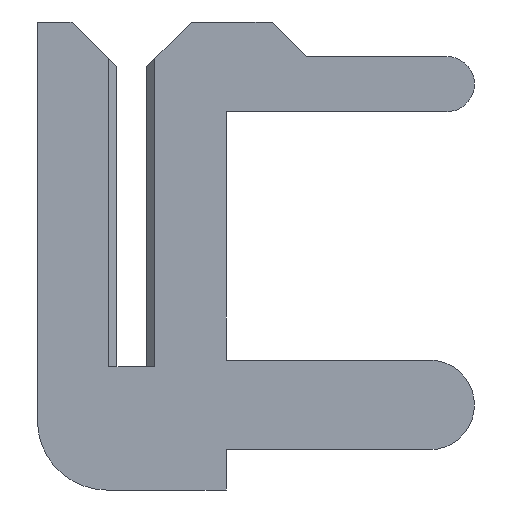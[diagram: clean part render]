
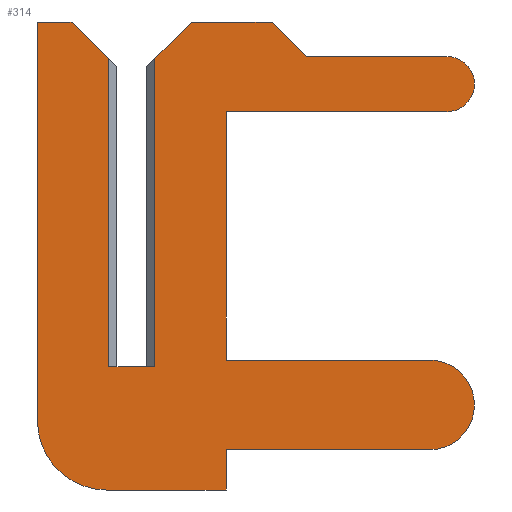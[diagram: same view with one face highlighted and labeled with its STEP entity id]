
A CAD part, left-side view. The second image highlights one B-rep face of the part: STEP entity #314.
In plain terms, the highlighted planar face has unit normal (-1, 0, 0).
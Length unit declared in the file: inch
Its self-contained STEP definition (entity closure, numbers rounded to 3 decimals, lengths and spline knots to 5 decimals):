
#5 = ORIENTED_EDGE ( 'NONE', *, *, #1200, .F. ) ;
#7 = VERTEX_POINT ( 'NONE', #64 ) ;
#8 = EDGE_CURVE ( 'NONE', #683, #844, #404, .T. ) ;
#40 = VECTOR ( 'NONE', #839, 39.37008 ) ;
#43 = AXIS2_PLACEMENT_3D ( 'NONE', #395, #286, #94 ) ;
#48 = CARTESIAN_POINT ( 'NONE',  ( -0.01, -0.137, 0.111 ) ) ;
#51 = VERTEX_POINT ( 'NONE', #527 ) ;
#52 = EDGE_CURVE ( 'NONE', #713, #859, #476, .T. ) ;
#58 = DIRECTION ( 'NONE',  ( 0., 0., 1. ) ) ;
#59 = VERTEX_POINT ( 'NONE', #336 ) ;
#64 = CARTESIAN_POINT ( 'NONE',  ( -0.01, -0.01, 0. ) ) ;
#67 = EDGE_CURVE ( 'NONE', #59, #7, #883, .T. ) ;
#69 = CARTESIAN_POINT ( 'NONE',  ( -0.01, -0.1295, 0.003 ) ) ;
#86 = LINE ( 'NONE', #69, #1009 ) ;
#94 = DIRECTION ( 'NONE',  ( 0., 0., 1. ) ) ;
#118 = EDGE_LOOP ( 'NONE', ( #1059, #1040, #791, #230, #5, #1042, #881, #497, #1221, #818, #893, #371, #251, #534, #278, #431, #1159, #1102, #756 ) ) ;
#146 = CARTESIAN_POINT ( 'NONE',  ( -0.01, -0.041, 0.111 ) ) ;
#148 = AXIS2_PLACEMENT_3D ( 'NONE', #1144, #942, #1112 ) ;
#156 = EDGE_CURVE ( 'NONE', #859, #778, #1106, .T. ) ;
#180 = CARTESIAN_POINT ( 'NONE',  ( -0.01, -0.041, -0.0535 ) ) ;
#208 = EDGE_CURVE ( 'NONE', #774, #328, #1032, .T. ) ;
#223 = VECTOR ( 'NONE', #699, 39.37008 ) ;
#230 = ORIENTED_EDGE ( 'NONE', *, *, #208, .T. ) ;
#237 = VECTOR ( 'NONE', #835, 39.37008 ) ;
#246 = VECTOR ( 'NONE', #58, 39.37008 ) ;
#251 = ORIENTED_EDGE ( 'NONE', *, *, #941, .F. ) ;
#257 = DIRECTION ( 'NONE',  ( 0., 0., 1. ) ) ;
#278 = ORIENTED_EDGE ( 'NONE', *, *, #156, .F. ) ;
#284 = CARTESIAN_POINT ( 'NONE',  ( -0.01, -0.041, 0.003 ) ) ;
#286 = DIRECTION ( 'NONE',  ( 1., 0., 0. ) ) ;
#287 = EDGE_CURVE ( 'NONE', #59, #1206, #653, .T. ) ;
#288 = CARTESIAN_POINT ( 'NONE',  ( -0.01, 0.0065, 0.1305 ) ) ;
#294 = VERTEX_POINT ( 'NONE', #284 ) ;
#307 = DIRECTION ( 'NONE',  ( 0., -1., 0. ) ) ;
#314 = ADVANCED_FACE ( 'NONE', ( #885 ), #937, .T. ) ;
#325 = CARTESIAN_POINT ( 'NONE',  ( -0.01, 0.0065, 0. ) ) ;
#328 = VERTEX_POINT ( 'NONE', #1034 ) ;
#333 = CARTESIAN_POINT ( 'NONE',  ( -0.01, 0.01, 0. ) ) ;
#336 = CARTESIAN_POINT ( 'NONE',  ( -0.01, -0.01, 0.134 ) ) ;
#346 = DIRECTION ( 'NONE',  ( 0., 0., -1. ) ) ;
#371 = ORIENTED_EDGE ( 'NONE', *, *, #519, .F. ) ;
#382 = DIRECTION ( 'NONE',  ( 0., -1., 0. ) ) ;
#395 = CARTESIAN_POINT ( 'NONE',  ( -0.01, -0.1295, -0.0165 ) ) ;
#404 = CIRCLE ( 'NONE', #1037, 0.03 ) ;
#419 = DIRECTION ( 'NONE',  ( 0., -1., 0. ) ) ;
#431 = ORIENTED_EDGE ( 'NONE', *, *, #52, .F. ) ;
#432 = CARTESIAN_POINT ( 'NONE',  ( -0.01, 0.011, -0.0235 ) ) ;
#433 = DIRECTION ( 'NONE',  ( 0., -1., 0. ) ) ;
#440 = CIRCLE ( 'NONE', #43, 0.0195 ) ;
#442 = CARTESIAN_POINT ( 'NONE',  ( -0.01, 0.041, 0.15 ) ) ;
#452 = EDGE_CURVE ( 'NONE', #680, #651, #915, .T. ) ;
#476 = CIRCLE ( 'NONE', #506, 0.012 ) ;
#482 = VECTOR ( 'NONE', #1038, 39.37008 ) ;
#483 = CARTESIAN_POINT ( 'NONE',  ( -0.01, -0.076, 0.135 ) ) ;
#485 = LINE ( 'NONE', #1148, #913 ) ;
#492 = LINE ( 'NONE', #442, #246 ) ;
#494 = VERTEX_POINT ( 'NONE', #975 ) ;
#497 = ORIENTED_EDGE ( 'NONE', *, *, #8, .F. ) ;
#506 = AXIS2_PLACEMENT_3D ( 'NONE', #716, #812, #257 ) ;
#519 = EDGE_CURVE ( 'NONE', #730, #51, #440, .T. ) ;
#520 = DIRECTION ( 'NONE',  ( 1., 0., 0. ) ) ;
#521 = CARTESIAN_POINT ( 'NONE',  ( -0.01, 0.041, -0.0235 ) ) ;
#525 = VERTEX_POINT ( 'NONE', #1132 ) ;
#527 = CARTESIAN_POINT ( 'NONE',  ( -0.01, -0.1295, -0.036 ) ) ;
#531 = CARTESIAN_POINT ( 'NONE',  ( -0.01, 0.026, 0.15 ) ) ;
#534 = ORIENTED_EDGE ( 'NONE', *, *, #599, .F. ) ;
#535 = VERTEX_POINT ( 'NONE', #1125 ) ;
#542 = LINE ( 'NONE', #858, #886 ) ;
#552 = LINE ( 'NONE', #180, #40 ) ;
#577 = CARTESIAN_POINT ( 'NONE',  ( -0.01, 0.011, -0.0535 ) ) ;
#591 = EDGE_CURVE ( 'NONE', #525, #683, #485, .T. ) ;
#599 = EDGE_CURVE ( 'NONE', #778, #294, #641, .T. ) ;
#611 = CARTESIAN_POINT ( 'NONE',  ( -0.01, -0.137, 0.135 ) ) ;
#632 = EDGE_CURVE ( 'NONE', #651, #713, #542, .T. ) ;
#641 = LINE ( 'NONE', #765, #869 ) ;
#651 = VERTEX_POINT ( 'NONE', #483 ) ;
#653 = LINE ( 'NONE', #1130, #482 ) ;
#665 = CARTESIAN_POINT ( 'NONE',  ( -0.01, -0.026, 0.15 ) ) ;
#670 = DIRECTION ( 'NONE',  ( 0., -0.707, -0.707 ) ) ;
#680 = VERTEX_POINT ( 'NONE', #1060 ) ;
#681 = EDGE_CURVE ( 'NONE', #1206, #680, #1070, .T. ) ;
#683 = VERTEX_POINT ( 'NONE', #577 ) ;
#686 = DIRECTION ( 'NONE',  ( 0., -0.707, -0.707 ) ) ;
#698 = CARTESIAN_POINT ( 'NONE',  ( -0.01, -0.076, 0.135 ) ) ;
#699 = DIRECTION ( 'NONE',  ( 0., 1., 0. ) ) ;
#704 = CARTESIAN_POINT ( 'NONE',  ( -0.01, -0.041, -0.036 ) ) ;
#707 = VECTOR ( 'NONE', #433, 39.37008 ) ;
#713 = VERTEX_POINT ( 'NONE', #611 ) ;
#716 = CARTESIAN_POINT ( 'NONE',  ( -0.01, -0.137, 0.123 ) ) ;
#723 = VERTEX_POINT ( 'NONE', #1185 ) ;
#730 = VERTEX_POINT ( 'NONE', #994 ) ;
#733 = CARTESIAN_POINT ( 'NONE',  ( -0.01, 0.01, -0.0235 ) ) ;
#736 = VECTOR ( 'NONE', #686, 39.37008 ) ;
#749 = EDGE_CURVE ( 'NONE', #51, #723, #973, .T. ) ;
#756 = ORIENTED_EDGE ( 'NONE', *, *, #681, .F. ) ;
#765 = CARTESIAN_POINT ( 'NONE',  ( -0.01, -0.041, 0.003 ) ) ;
#774 = VERTEX_POINT ( 'NONE', #333 ) ;
#778 = VERTEX_POINT ( 'NONE', #146 ) ;
#789 = VECTOR ( 'NONE', #346, 39.37008 ) ;
#791 = ORIENTED_EDGE ( 'NONE', *, *, #811, .F. ) ;
#801 = LINE ( 'NONE', #288, #985 ) ;
#805 = DIRECTION ( 'NONE',  ( 0., 0., 1. ) ) ;
#811 = EDGE_CURVE ( 'NONE', #774, #7, #1056, .T. ) ;
#812 = DIRECTION ( 'NONE',  ( 1., 0., 0. ) ) ;
#818 = ORIENTED_EDGE ( 'NONE', *, *, #1177, .F. ) ;
#823 = DIRECTION ( 'NONE',  ( 0., -1., 0. ) ) ;
#833 = EDGE_CURVE ( 'NONE', #494, #535, #1216, .T. ) ;
#835 = DIRECTION ( 'NONE',  ( 0., 0., 1. ) ) ;
#839 = DIRECTION ( 'NONE',  ( 0., 0., -1. ) ) ;
#844 = VERTEX_POINT ( 'NONE', #521 ) ;
#849 = VECTOR ( 'NONE', #307, 39.37008 ) ;
#858 = CARTESIAN_POINT ( 'NONE',  ( -0.01, -0.137, 0.135 ) ) ;
#859 = VERTEX_POINT ( 'NONE', #48 ) ;
#869 = VECTOR ( 'NONE', #1045, 39.37008 ) ;
#881 = ORIENTED_EDGE ( 'NONE', *, *, #1047, .F. ) ;
#883 = LINE ( 'NONE', #907, #789 ) ;
#885 = FACE_OUTER_BOUND ( 'NONE', #118, .T. ) ;
#886 = VECTOR ( 'NONE', #382, 39.37008 ) ;
#893 = ORIENTED_EDGE ( 'NONE', *, *, #749, .F. ) ;
#907 = CARTESIAN_POINT ( 'NONE',  ( -0.01, -0.01, 0.15 ) ) ;
#913 = VECTOR ( 'NONE', #1068, 39.37008 ) ;
#915 = LINE ( 'NONE', #698, #736 ) ;
#920 = CARTESIAN_POINT ( 'NONE',  ( -0.01, -0.041, 0.111 ) ) ;
#937 = PLANE ( 'NONE',  #148 ) ;
#941 = EDGE_CURVE ( 'NONE', #294, #730, #86, .T. ) ;
#942 = DIRECTION ( 'NONE',  ( -1., 0., 0. ) ) ;
#968 = VECTOR ( 'NONE', #1117, 39.37008 ) ;
#973 = LINE ( 'NONE', #704, #223 ) ;
#975 = CARTESIAN_POINT ( 'NONE',  ( -0.01, 0.041, 0.15 ) ) ;
#985 = VECTOR ( 'NONE', #670, 39.37008 ) ;
#994 = CARTESIAN_POINT ( 'NONE',  ( -0.01, -0.1295, 0.003 ) ) ;
#1009 = VECTOR ( 'NONE', #823, 39.37008 ) ;
#1022 = VECTOR ( 'NONE', #419, 39.37008 ) ;
#1032 = LINE ( 'NONE', #733, #237 ) ;
#1034 = CARTESIAN_POINT ( 'NONE',  ( -0.01, 0.01, 0.134 ) ) ;
#1037 = AXIS2_PLACEMENT_3D ( 'NONE', #432, #520, #805 ) ;
#1038 = DIRECTION ( 'NONE',  ( 0., -0.707, 0.707 ) ) ;
#1039 = CARTESIAN_POINT ( 'NONE',  ( -0.01, -0.026, 0.15 ) ) ;
#1040 = ORIENTED_EDGE ( 'NONE', *, *, #67, .T. ) ;
#1042 = ORIENTED_EDGE ( 'NONE', *, *, #833, .F. ) ;
#1045 = DIRECTION ( 'NONE',  ( 0., 0., -1. ) ) ;
#1047 = EDGE_CURVE ( 'NONE', #844, #494, #492, .T. ) ;
#1056 = LINE ( 'NONE', #325, #1022 ) ;
#1059 = ORIENTED_EDGE ( 'NONE', *, *, #287, .F. ) ;
#1060 = CARTESIAN_POINT ( 'NONE',  ( -0.01, -0.061, 0.15 ) ) ;
#1068 = DIRECTION ( 'NONE',  ( 0., 1., 0. ) ) ;
#1070 = LINE ( 'NONE', #665, #849 ) ;
#1102 = ORIENTED_EDGE ( 'NONE', *, *, #452, .F. ) ;
#1106 = LINE ( 'NONE', #920, #968 ) ;
#1112 = DIRECTION ( 'NONE',  ( 0., 0., 1. ) ) ;
#1117 = DIRECTION ( 'NONE',  ( 0., 1., 0. ) ) ;
#1125 = CARTESIAN_POINT ( 'NONE',  ( -0.01, 0.026, 0.15 ) ) ;
#1130 = CARTESIAN_POINT ( 'NONE',  ( -0.01, -0.0065, 0.1305 ) ) ;
#1132 = CARTESIAN_POINT ( 'NONE',  ( -0.01, -0.041, -0.0535 ) ) ;
#1144 = CARTESIAN_POINT ( 'NONE',  ( -0.01, 0.011, -0.0235 ) ) ;
#1148 = CARTESIAN_POINT ( 'NONE',  ( -0.01, 0.011, -0.0535 ) ) ;
#1159 = ORIENTED_EDGE ( 'NONE', *, *, #632, .F. ) ;
#1177 = EDGE_CURVE ( 'NONE', #723, #525, #552, .T. ) ;
#1185 = CARTESIAN_POINT ( 'NONE',  ( -0.01, -0.041, -0.036 ) ) ;
#1200 = EDGE_CURVE ( 'NONE', #535, #328, #801, .T. ) ;
#1206 = VERTEX_POINT ( 'NONE', #1039 ) ;
#1216 = LINE ( 'NONE', #531, #707 ) ;
#1221 = ORIENTED_EDGE ( 'NONE', *, *, #591, .F. ) ;
